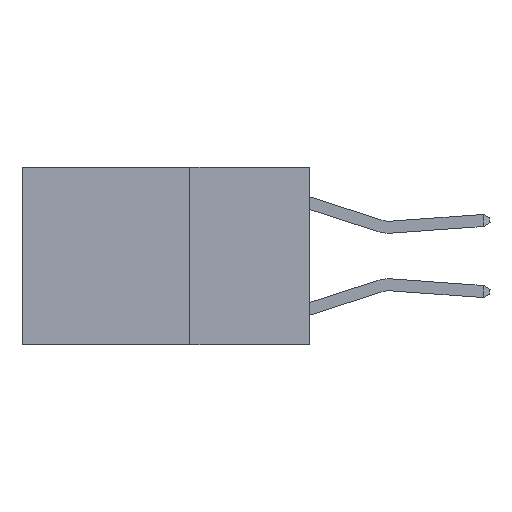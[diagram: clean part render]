
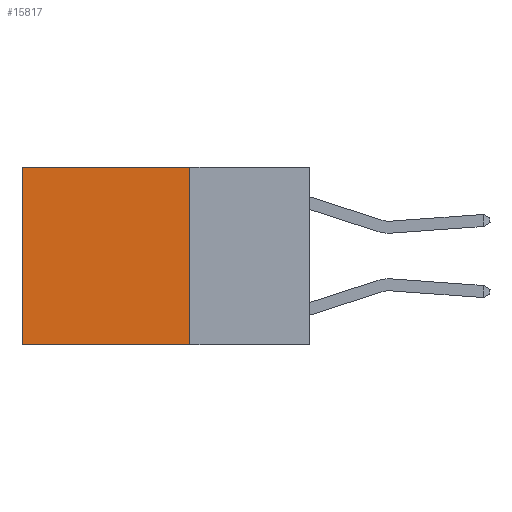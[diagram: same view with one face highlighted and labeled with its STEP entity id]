
A CAD part, left-side view. The second image highlights one B-rep face of the part: STEP entity #15817.
In plain terms, the highlighted planar face has unit normal (-1, 0, 0).
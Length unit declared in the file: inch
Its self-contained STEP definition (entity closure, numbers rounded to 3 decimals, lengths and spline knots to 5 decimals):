
#472 = LINE ( 'NONE', #2703, #5460 ) ;
#870 = DIRECTION ( 'NONE',  ( 0., 1., 0. ) ) ;
#1324 = CARTESIAN_POINT ( 'NONE',  ( 0.2625, 0.25, 0. ) ) ;
#1546 = VERTEX_POINT ( 'NONE', #7157 ) ;
#1597 = FACE_OUTER_BOUND ( 'NONE', #18479, .T. ) ;
#1640 = CARTESIAN_POINT ( 'NONE',  ( 0.2625, 0.6, 0. ) ) ;
#2703 = CARTESIAN_POINT ( 'NONE',  ( 0.2625, 0.25, -0.37 ) ) ;
#3031 = AXIS2_PLACEMENT_3D ( 'NONE', #15112, #18931, #3410 ) ;
#3158 = LINE ( 'NONE', #14981, #17300 ) ;
#3410 = DIRECTION ( 'NONE',  ( 0., 0., -1. ) ) ;
#4059 = CARTESIAN_POINT ( 'NONE',  ( 0.2625, 0.6, 0. ) ) ;
#4091 = CARTESIAN_POINT ( 'NONE',  ( 0.2625, 0.25, 0. ) ) ;
#4093 = VERTEX_POINT ( 'NONE', #1324 ) ;
#5078 = VERTEX_POINT ( 'NONE', #1640 ) ;
#5460 = VECTOR ( 'NONE', #870, 39.37008 ) ;
#6982 = CARTESIAN_POINT ( 'NONE',  ( 0.2625, 0.6, -0.37 ) ) ;
#7157 = CARTESIAN_POINT ( 'NONE',  ( 0.2625, 0.25, -0.37 ) ) ;
#7345 = ORIENTED_EDGE ( 'NONE', *, *, #21478, .T. ) ;
#8303 = ORIENTED_EDGE ( 'NONE', *, *, #25204, .F. ) ;
#8739 = ORIENTED_EDGE ( 'NONE', *, *, #17685, .F. ) ;
#9203 = VECTOR ( 'NONE', #15535, 39.37008 ) ;
#12187 = LINE ( 'NONE', #4091, #9203 ) ;
#14444 = ORIENTED_EDGE ( 'NONE', *, *, #18320, .T. ) ;
#14827 = VERTEX_POINT ( 'NONE', #6982 ) ;
#14981 = CARTESIAN_POINT ( 'NONE',  ( 0.2625, 0.25, 0. ) ) ;
#15112 = CARTESIAN_POINT ( 'NONE',  ( 0.2625, 0.25, 0. ) ) ;
#15535 = DIRECTION ( 'NONE',  ( 0., 0., -1. ) ) ;
#15817 = ADVANCED_FACE ( 'NONE', ( #1597 ), #25213, .F. ) ;
#17300 = VECTOR ( 'NONE', #25195, 39.37008 ) ;
#17685 = EDGE_CURVE ( 'NONE', #4093, #1546, #12187, .T. ) ;
#18320 = EDGE_CURVE ( 'NONE', #5078, #14827, #20204, .T. ) ;
#18479 = EDGE_LOOP ( 'NONE', ( #14444, #8303, #8739, #7345 ) ) ;
#18931 = DIRECTION ( 'NONE',  ( 1., 0., 0. ) ) ;
#20204 = LINE ( 'NONE', #4059, #23532 ) ;
#21478 = EDGE_CURVE ( 'NONE', #4093, #5078, #3158, .T. ) ;
#23532 = VECTOR ( 'NONE', #23921, 39.37008 ) ;
#23921 = DIRECTION ( 'NONE',  ( 0., 0., -1. ) ) ;
#25195 = DIRECTION ( 'NONE',  ( 0., 1., 0. ) ) ;
#25204 = EDGE_CURVE ( 'NONE', #1546, #14827, #472, .T. ) ;
#25213 = PLANE ( 'NONE',  #3031 ) ;
